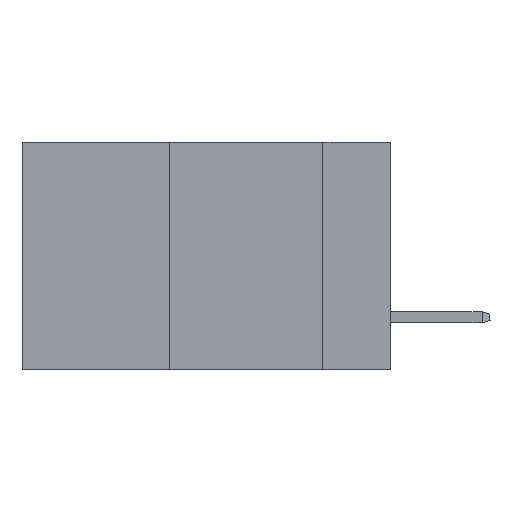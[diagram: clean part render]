
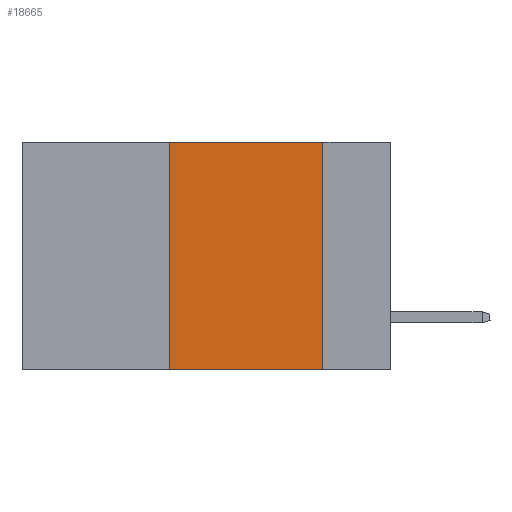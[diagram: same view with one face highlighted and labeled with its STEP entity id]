
A CAD part, left-side view. The second image highlights one B-rep face of the part: STEP entity #18665.
In plain terms, the highlighted planar face has unit normal (-1, 0, 0).
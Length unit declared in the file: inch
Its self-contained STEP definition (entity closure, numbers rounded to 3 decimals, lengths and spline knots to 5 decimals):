
#758 = CARTESIAN_POINT ( 'NONE',  ( 0., 0.11, -0.37 ) ) ;
#1381 = FACE_OUTER_BOUND ( 'NONE', #5981, .T. ) ;
#2567 = ORIENTED_EDGE ( 'NONE', *, *, #12380, .F. ) ;
#2947 = CARTESIAN_POINT ( 'NONE',  ( 0., 0.36, -0.37 ) ) ;
#5981 = EDGE_LOOP ( 'NONE', ( #2567, #17813, #14895, #19763 ) ) ;
#7447 = VECTOR ( 'NONE', #17498, 39.37008 ) ;
#8455 = DIRECTION ( 'NONE',  ( 0., 0., -1. ) ) ;
#8519 = VERTEX_POINT ( 'NONE', #2947 ) ;
#9137 = PLANE ( 'NONE',  #17031 ) ;
#11511 = DIRECTION ( 'NONE',  ( 0., 0., -1. ) ) ;
#12380 = EDGE_CURVE ( 'NONE', #26198, #27121, #13473, .T. ) ;
#13473 = LINE ( 'NONE', #19913, #25659 ) ;
#14167 = LINE ( 'NONE', #19220, #16863 ) ;
#14396 = LINE ( 'NONE', #25664, #17119 ) ;
#14895 = ORIENTED_EDGE ( 'NONE', *, *, #23142, .F. ) ;
#15890 = EDGE_CURVE ( 'NONE', #22348, #26198, #14396, .T. ) ;
#16863 = VECTOR ( 'NONE', #27742, 39.37008 ) ;
#17031 = AXIS2_PLACEMENT_3D ( 'NONE', #24263, #18002, #11511 ) ;
#17119 = VECTOR ( 'NONE', #17149, 39.37008 ) ;
#17149 = DIRECTION ( 'NONE',  ( 0., -1., 0. ) ) ;
#17498 = DIRECTION ( 'NONE',  ( 0., -1., 0. ) ) ;
#17684 = CARTESIAN_POINT ( 'NONE',  ( 0., 0.6, -0.37 ) ) ;
#17813 = ORIENTED_EDGE ( 'NONE', *, *, #15890, .F. ) ;
#18002 = DIRECTION ( 'NONE',  ( 1., 0., 0. ) ) ;
#18665 = ADVANCED_FACE ( 'NONE', ( #1381 ), #9137, .F. ) ;
#19220 = CARTESIAN_POINT ( 'NONE',  ( 0., 0.36, 0. ) ) ;
#19763 = ORIENTED_EDGE ( 'NONE', *, *, #26424, .T. ) ;
#19913 = CARTESIAN_POINT ( 'NONE',  ( 0., 0.11, 0. ) ) ;
#20279 = CARTESIAN_POINT ( 'NONE',  ( 0., 0.36, 0. ) ) ;
#22348 = VERTEX_POINT ( 'NONE', #20279 ) ;
#23142 = EDGE_CURVE ( 'NONE', #8519, #22348, #14167, .T. ) ;
#24263 = CARTESIAN_POINT ( 'NONE',  ( 0., 0.6, 0. ) ) ;
#24351 = LINE ( 'NONE', #17684, #7447 ) ;
#25659 = VECTOR ( 'NONE', #8455, 39.37008 ) ;
#25664 = CARTESIAN_POINT ( 'NONE',  ( 0., 0.6, 0. ) ) ;
#26198 = VERTEX_POINT ( 'NONE', #27063 ) ;
#26424 = EDGE_CURVE ( 'NONE', #8519, #27121, #24351, .T. ) ;
#27063 = CARTESIAN_POINT ( 'NONE',  ( 0., 0.11, 0. ) ) ;
#27121 = VERTEX_POINT ( 'NONE', #758 ) ;
#27742 = DIRECTION ( 'NONE',  ( 0., 0., 1. ) ) ;
